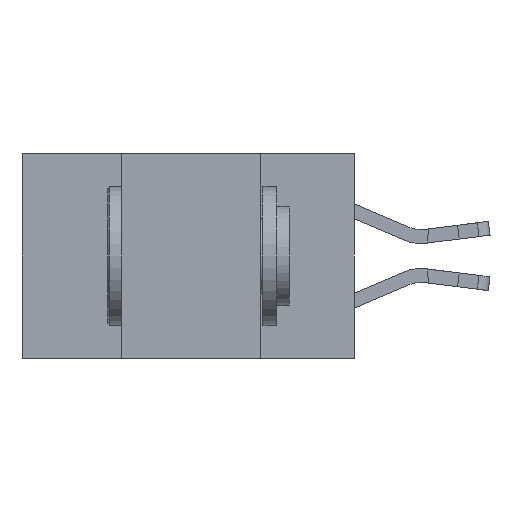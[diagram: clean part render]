
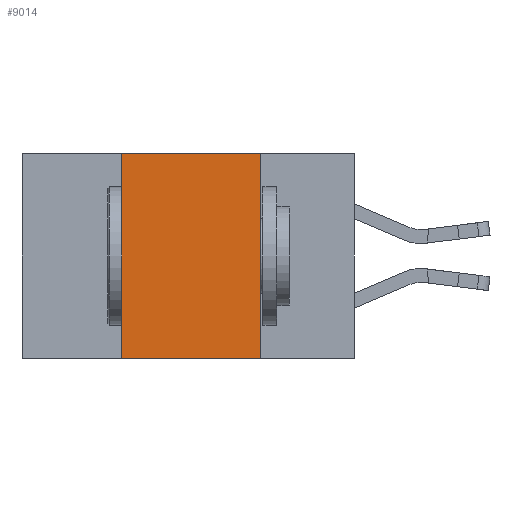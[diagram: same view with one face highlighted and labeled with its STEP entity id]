
A CAD part, left-side view. The second image highlights one B-rep face of the part: STEP entity #9014.
In plain terms, the highlighted planar face has unit normal (-1, 0, 0).
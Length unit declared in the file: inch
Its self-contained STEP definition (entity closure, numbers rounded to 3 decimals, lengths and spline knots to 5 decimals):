
#60 = VECTOR ( 'NONE', #8839, 39.37008 ) ;
#764 = CARTESIAN_POINT ( 'NONE',  ( 0., 0.17, -0.37 ) ) ;
#860 = ORIENTED_EDGE ( 'NONE', *, *, #9313, .F. ) ;
#1067 = CARTESIAN_POINT ( 'NONE',  ( 0., 0.6, 0. ) ) ;
#1328 = CARTESIAN_POINT ( 'NONE',  ( 0., 0.42, 0. ) ) ;
#1428 = ORIENTED_EDGE ( 'NONE', *, *, #6674, .F. ) ;
#2531 = DIRECTION ( 'NONE',  ( 0., -1., 0. ) ) ;
#2617 = CARTESIAN_POINT ( 'NONE',  ( 0., 0.6, 0. ) ) ;
#3672 = EDGE_LOOP ( 'NONE', ( #860, #1428, #3808, #6806 ) ) ;
#3691 = VERTEX_POINT ( 'NONE', #6798 ) ;
#3784 = VERTEX_POINT ( 'NONE', #8915 ) ;
#3808 = ORIENTED_EDGE ( 'NONE', *, *, #5695, .F. ) ;
#4181 = VERTEX_POINT ( 'NONE', #764 ) ;
#4217 = DIRECTION ( 'NONE',  ( 0., 0., -1. ) ) ;
#5034 = LINE ( 'NONE', #11200, #10813 ) ;
#5189 = AXIS2_PLACEMENT_3D ( 'NONE', #2617, #6148, #7275 ) ;
#5695 = EDGE_CURVE ( 'NONE', #3691, #7656, #5034, .T. ) ;
#6017 = CARTESIAN_POINT ( 'NONE',  ( 0., 0.17, -0.37 ) ) ;
#6148 = DIRECTION ( 'NONE',  ( 1., 0., 0. ) ) ;
#6674 = EDGE_CURVE ( 'NONE', #7656, #3784, #10374, .T. ) ;
#6798 = CARTESIAN_POINT ( 'NONE',  ( 0., 0.42, -0.37 ) ) ;
#6806 = ORIENTED_EDGE ( 'NONE', *, *, #8059, .T. ) ;
#7275 = DIRECTION ( 'NONE',  ( 0., 0., -1. ) ) ;
#7656 = VERTEX_POINT ( 'NONE', #1328 ) ;
#7844 = VECTOR ( 'NONE', #4217, 39.37008 ) ;
#7848 = LINE ( 'NONE', #6017, #7844 ) ;
#8059 = EDGE_CURVE ( 'NONE', #3691, #4181, #9665, .T. ) ;
#8394 = VECTOR ( 'NONE', #2531, 39.37008 ) ;
#8670 = DIRECTION ( 'NONE',  ( 0., 0., 1. ) ) ;
#8839 = DIRECTION ( 'NONE',  ( 0., -1., 0. ) ) ;
#8915 = CARTESIAN_POINT ( 'NONE',  ( 0., 0.17, 0. ) ) ;
#8928 = FACE_OUTER_BOUND ( 'NONE', #3672, .T. ) ;
#9014 = ADVANCED_FACE ( 'NONE', ( #8928 ), #9813, .F. ) ;
#9313 = EDGE_CURVE ( 'NONE', #3784, #4181, #7848, .T. ) ;
#9665 = LINE ( 'NONE', #10327, #8394 ) ;
#9813 = PLANE ( 'NONE',  #5189 ) ;
#10327 = CARTESIAN_POINT ( 'NONE',  ( 0., 0.6, -0.37 ) ) ;
#10374 = LINE ( 'NONE', #1067, #60 ) ;
#10813 = VECTOR ( 'NONE', #8670, 39.37008 ) ;
#11200 = CARTESIAN_POINT ( 'NONE',  ( 0., 0.42, -0.37 ) ) ;
